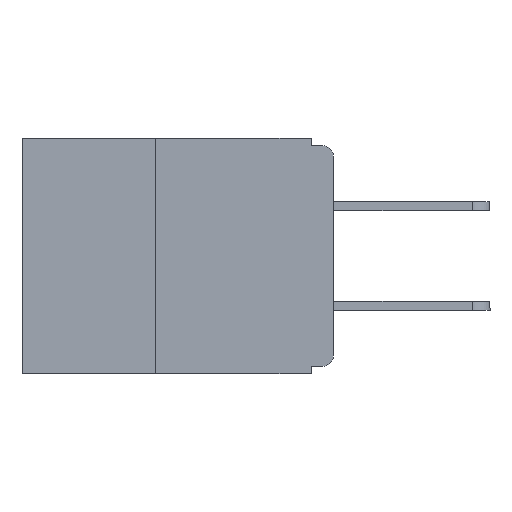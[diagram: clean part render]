
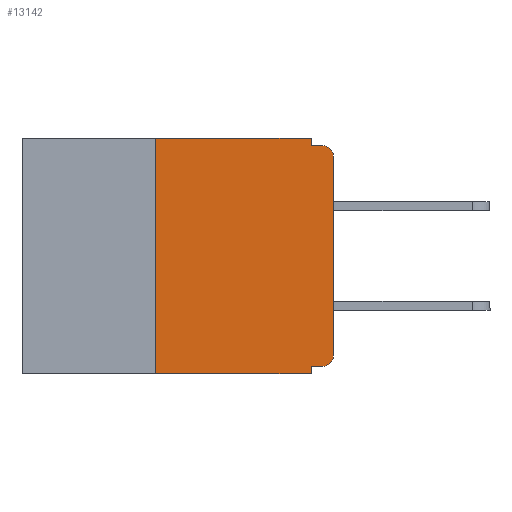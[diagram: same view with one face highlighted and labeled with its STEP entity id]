
A CAD part, left-side view. The second image highlights one B-rep face of the part: STEP entity #13142.
In plain terms, the highlighted planar face has unit normal (-1, 0, 0).
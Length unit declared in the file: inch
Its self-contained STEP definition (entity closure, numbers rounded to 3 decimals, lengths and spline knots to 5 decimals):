
#172 = CARTESIAN_POINT ( 'NONE',  ( 0., 0.015, -0.01 ) ) ;
#403 = EDGE_CURVE ( 'NONE', #13971, #12026, #2479, .T. ) ;
#511 = VERTEX_POINT ( 'NONE', #13681 ) ;
#805 = ORIENTED_EDGE ( 'NONE', *, *, #13868, .F. ) ;
#1058 = ORIENTED_EDGE ( 'NONE', *, *, #10749, .F. ) ;
#1092 = LINE ( 'NONE', #6759, #3497 ) ;
#1113 = DIRECTION ( 'NONE',  ( 1., 0., 0. ) ) ;
#1448 = CARTESIAN_POINT ( 'NONE',  ( 0., 0.031, -0.32 ) ) ;
#1489 = CARTESIAN_POINT ( 'NONE',  ( 0., 0.015, -0.025 ) ) ;
#1626 = CARTESIAN_POINT ( 'NONE',  ( 0., 0.25, -0.33 ) ) ;
#1850 = CARTESIAN_POINT ( 'NONE',  ( 0., 0.437, 0. ) ) ;
#2305 = DIRECTION ( 'NONE',  ( 0., 0., -1. ) ) ;
#2378 = DIRECTION ( 'NONE',  ( 0., -1., 0. ) ) ;
#2479 = LINE ( 'NONE', #1850, #9296 ) ;
#2638 = DIRECTION ( 'NONE',  ( 0., 0., -1. ) ) ;
#2676 = ORIENTED_EDGE ( 'NONE', *, *, #6668, .F. ) ;
#2706 = ORIENTED_EDGE ( 'NONE', *, *, #403, .F. ) ;
#2770 = CIRCLE ( 'NONE', #4613, 0.015 ) ;
#2800 = LINE ( 'NONE', #4801, #11609 ) ;
#2920 = CARTESIAN_POINT ( 'NONE',  ( 0., 0., -0.01 ) ) ;
#2952 = DIRECTION ( 'NONE',  ( 0., -1., 0. ) ) ;
#3262 = ORIENTED_EDGE ( 'NONE', *, *, #6851, .F. ) ;
#3467 = LINE ( 'NONE', #13588, #5617 ) ;
#3497 = VECTOR ( 'NONE', #12579, 39.37008 ) ;
#4052 = DIRECTION ( 'NONE',  ( 0., 0., 1. ) ) ;
#4283 = AXIS2_PLACEMENT_3D ( 'NONE', #7160, #1113, #9503 ) ;
#4497 = EDGE_CURVE ( 'NONE', #5013, #10600, #2770, .T. ) ;
#4613 = AXIS2_PLACEMENT_3D ( 'NONE', #8354, #8147, #8051 ) ;
#4801 = CARTESIAN_POINT ( 'NONE',  ( 0., 0.031, 0. ) ) ;
#4874 = VERTEX_POINT ( 'NONE', #9166 ) ;
#5013 = VERTEX_POINT ( 'NONE', #6370 ) ;
#5250 = ORIENTED_EDGE ( 'NONE', *, *, #14732, .F. ) ;
#5429 = VECTOR ( 'NONE', #2952, 39.37008 ) ;
#5617 = VECTOR ( 'NONE', #10129, 39.37008 ) ;
#5837 = ORIENTED_EDGE ( 'NONE', *, *, #4497, .T. ) ;
#5934 = DIRECTION ( 'NONE',  ( 0., -1., 0. ) ) ;
#6014 = VECTOR ( 'NONE', #9992, 39.37008 ) ;
#6027 = VECTOR ( 'NONE', #4052, 39.37008 ) ;
#6370 = CARTESIAN_POINT ( 'NONE',  ( 0., 0.015, -0.32 ) ) ;
#6408 = LINE ( 'NONE', #8844, #6027 ) ;
#6668 = EDGE_CURVE ( 'NONE', #10971, #7949, #11335, .T. ) ;
#6759 = CARTESIAN_POINT ( 'NONE',  ( 0., 0., -0.32 ) ) ;
#6851 = EDGE_CURVE ( 'NONE', #9091, #511, #3467, .T. ) ;
#7160 = CARTESIAN_POINT ( 'NONE',  ( 0., 0.437, 0. ) ) ;
#7193 = CARTESIAN_POINT ( 'NONE',  ( 0., 0.25, -0.33 ) ) ;
#7324 = ORIENTED_EDGE ( 'NONE', *, *, #15198, .T. ) ;
#7358 = LINE ( 'NONE', #9616, #13526 ) ;
#7949 = VERTEX_POINT ( 'NONE', #172 ) ;
#8051 = DIRECTION ( 'NONE',  ( 0., 0., -1. ) ) ;
#8147 = DIRECTION ( 'NONE',  ( -1., 0., 0. ) ) ;
#8354 = CARTESIAN_POINT ( 'NONE',  ( 0., 0.015, -0.305 ) ) ;
#8844 = CARTESIAN_POINT ( 'NONE',  ( 0., 0., 0. ) ) ;
#9091 = VERTEX_POINT ( 'NONE', #1448 ) ;
#9166 = CARTESIAN_POINT ( 'NONE',  ( 0., 0., -0.025 ) ) ;
#9296 = VECTOR ( 'NONE', #5934, 39.37008 ) ;
#9412 = ORIENTED_EDGE ( 'NONE', *, *, #10080, .T. ) ;
#9503 = DIRECTION ( 'NONE',  ( 0., 0., -1. ) ) ;
#9616 = CARTESIAN_POINT ( 'NONE',  ( 0., 0.437, -0.33 ) ) ;
#9804 = FACE_OUTER_BOUND ( 'NONE', #13502, .T. ) ;
#9857 = DIRECTION ( 'NONE',  ( -1., 0., 0. ) ) ;
#9965 = EDGE_CURVE ( 'NONE', #11147, #511, #7358, .T. ) ;
#9992 = DIRECTION ( 'NONE',  ( 0., 0., 1. ) ) ;
#10080 = EDGE_CURVE ( 'NONE', #4874, #7949, #12089, .T. ) ;
#10129 = DIRECTION ( 'NONE',  ( 0., 0., -1. ) ) ;
#10600 = VERTEX_POINT ( 'NONE', #12053 ) ;
#10749 = EDGE_CURVE ( 'NONE', #11147, #13971, #12249, .T. ) ;
#10962 = ORIENTED_EDGE ( 'NONE', *, *, #9965, .T. ) ;
#10971 = VERTEX_POINT ( 'NONE', #12655 ) ;
#11133 = AXIS2_PLACEMENT_3D ( 'NONE', #1489, #9857, #2638 ) ;
#11147 = VERTEX_POINT ( 'NONE', #7193 ) ;
#11335 = LINE ( 'NONE', #2920, #5429 ) ;
#11609 = VECTOR ( 'NONE', #2305, 39.37008 ) ;
#12026 = VERTEX_POINT ( 'NONE', #14574 ) ;
#12053 = CARTESIAN_POINT ( 'NONE',  ( 0., 0., -0.305 ) ) ;
#12089 = CIRCLE ( 'NONE', #11133, 0.015 ) ;
#12249 = LINE ( 'NONE', #1626, #6014 ) ;
#12579 = DIRECTION ( 'NONE',  ( 0., 1., 0. ) ) ;
#12655 = CARTESIAN_POINT ( 'NONE',  ( 0., 0.031, -0.01 ) ) ;
#13142 = ADVANCED_FACE ( 'NONE', ( #9804 ), #15252, .F. ) ;
#13502 = EDGE_LOOP ( 'NONE', ( #7324, #9412, #2676, #805, #2706, #1058, #10962, #3262, #5250, #5837 ) ) ;
#13526 = VECTOR ( 'NONE', #2378, 39.37008 ) ;
#13588 = CARTESIAN_POINT ( 'NONE',  ( 0., 0.031, -0.33 ) ) ;
#13681 = CARTESIAN_POINT ( 'NONE',  ( 0., 0.031, -0.33 ) ) ;
#13868 = EDGE_CURVE ( 'NONE', #12026, #10971, #2800, .T. ) ;
#13971 = VERTEX_POINT ( 'NONE', #14840 ) ;
#14574 = CARTESIAN_POINT ( 'NONE',  ( 0., 0.031, 0. ) ) ;
#14732 = EDGE_CURVE ( 'NONE', #5013, #9091, #1092, .T. ) ;
#14840 = CARTESIAN_POINT ( 'NONE',  ( 0., 0.25, 0. ) ) ;
#15198 = EDGE_CURVE ( 'NONE', #10600, #4874, #6408, .T. ) ;
#15252 = PLANE ( 'NONE',  #4283 ) ;
